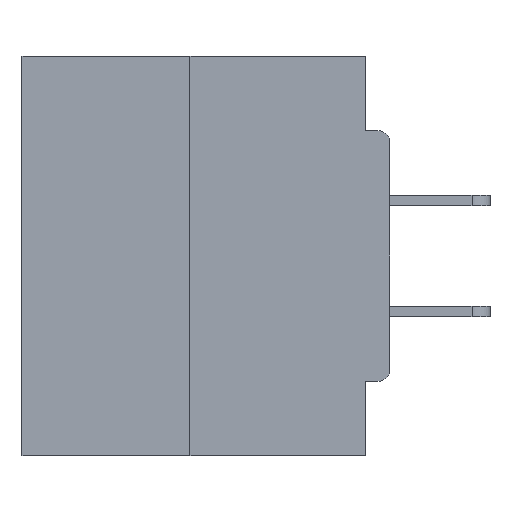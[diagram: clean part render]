
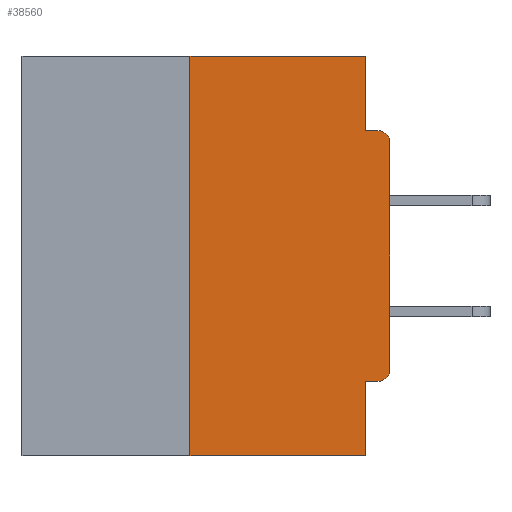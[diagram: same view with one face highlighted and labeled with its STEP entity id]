
A CAD part, left-side view. The second image highlights one B-rep face of the part: STEP entity #38560.
In plain terms, the highlighted planar face has unit normal (-1, 0, 0).
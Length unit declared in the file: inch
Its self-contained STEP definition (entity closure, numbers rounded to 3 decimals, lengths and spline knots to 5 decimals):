
#1169 = VERTEX_POINT ( 'NONE', #15668 ) ;
#1440 = CARTESIAN_POINT ( 'NONE',  ( 0., 0.25, 0. ) ) ;
#1769 = ORIENTED_EDGE ( 'NONE', *, *, #43550, .T. ) ;
#1906 = ORIENTED_EDGE ( 'NONE', *, *, #11319, .F. ) ;
#2708 = EDGE_CURVE ( 'NONE', #27769, #8198, #40876, .T. ) ;
#2900 = EDGE_CURVE ( 'NONE', #39610, #29801, #35509, .T. ) ;
#3965 = CARTESIAN_POINT ( 'NONE',  ( 0., 0.031, 0. ) ) ;
#4044 = DIRECTION ( 'NONE',  ( 1., 0., 0. ) ) ;
#4842 = LINE ( 'NONE', #8474, #19387 ) ;
#5030 = CARTESIAN_POINT ( 'NONE',  ( 0., 0.031, -0.5 ) ) ;
#5822 = VECTOR ( 'NONE', #8052, 39.37008 ) ;
#5872 = VERTEX_POINT ( 'NONE', #31267 ) ;
#6725 = EDGE_CURVE ( 'NONE', #26893, #35345, #37478, .T. ) ;
#8022 = DIRECTION ( 'NONE',  ( -1., 0., 0. ) ) ;
#8052 = DIRECTION ( 'NONE',  ( 0., 0., 1. ) ) ;
#8198 = VERTEX_POINT ( 'NONE', #33186 ) ;
#8277 = AXIS2_PLACEMENT_3D ( 'NONE', #28450, #4044, #28293 ) ;
#8474 = CARTESIAN_POINT ( 'NONE',  ( 0., 0.25, 0. ) ) ;
#8538 = VECTOR ( 'NONE', #15421, 39.37008 ) ;
#8597 = AXIS2_PLACEMENT_3D ( 'NONE', #35478, #8022, #11481 ) ;
#9036 = ORIENTED_EDGE ( 'NONE', *, *, #43108, .F. ) ;
#9143 = ORIENTED_EDGE ( 'NONE', *, *, #37754, .T. ) ;
#9298 = DIRECTION ( 'NONE',  ( 0., -1., 0. ) ) ;
#9304 = LINE ( 'NONE', #9726, #37368 ) ;
#9726 = CARTESIAN_POINT ( 'NONE',  ( 0., 0.46, -0.5 ) ) ;
#11319 = EDGE_CURVE ( 'NONE', #25590, #27769, #13968, .T. ) ;
#11481 = DIRECTION ( 'NONE',  ( 0., 0., -1. ) ) ;
#11743 = CARTESIAN_POINT ( 'NONE',  ( 0., 0.031, -0.4065 ) ) ;
#13191 = EDGE_CURVE ( 'NONE', #25590, #39610, #21374, .T. ) ;
#13324 = VECTOR ( 'NONE', #18516, 39.37008 ) ;
#13517 = DIRECTION ( 'NONE',  ( 0., 1., 0. ) ) ;
#13968 = LINE ( 'NONE', #31444, #34471 ) ;
#15421 = DIRECTION ( 'NONE',  ( 0., 0., -1. ) ) ;
#15668 = CARTESIAN_POINT ( 'NONE',  ( 0., 0.25, -0.5 ) ) ;
#16754 = EDGE_CURVE ( 'NONE', #5872, #30201, #39963, .T. ) ;
#16785 = CARTESIAN_POINT ( 'NONE',  ( 0., 0.015, -0.4065 ) ) ;
#17916 = PLANE ( 'NONE',  #8277 ) ;
#18516 = DIRECTION ( 'NONE',  ( 0., 0., -1. ) ) ;
#18864 = DIRECTION ( 'NONE',  ( 0., 0., 1. ) ) ;
#18934 = FACE_OUTER_BOUND ( 'NONE', #24641, .T. ) ;
#19387 = VECTOR ( 'NONE', #18864, 39.37008 ) ;
#21374 = CIRCLE ( 'NONE', #8597, 0.015 ) ;
#22225 = DIRECTION ( 'NONE',  ( 0., -1., 0. ) ) ;
#23190 = ORIENTED_EDGE ( 'NONE', *, *, #6725, .F. ) ;
#23720 = CARTESIAN_POINT ( 'NONE',  ( 0., 0.015, -0.1085 ) ) ;
#24641 = EDGE_LOOP ( 'NONE', ( #23190, #32181, #9143, #34505, #1906, #27550, #33647, #1769, #42073, #9036 ) ) ;
#24978 = CARTESIAN_POINT ( 'NONE',  ( 0., 0.46, 0. ) ) ;
#25590 = VERTEX_POINT ( 'NONE', #16785 ) ;
#26653 = VECTOR ( 'NONE', #31737, 39.37008 ) ;
#26893 = VERTEX_POINT ( 'NONE', #1440 ) ;
#27550 = ORIENTED_EDGE ( 'NONE', *, *, #13191, .T. ) ;
#27769 = VERTEX_POINT ( 'NONE', #11743 ) ;
#28293 = DIRECTION ( 'NONE',  ( 0., 0., -1. ) ) ;
#28450 = CARTESIAN_POINT ( 'NONE',  ( 0., 0.46, 0. ) ) ;
#28613 = AXIS2_PLACEMENT_3D ( 'NONE', #23720, #39744, #34315 ) ;
#28708 = CARTESIAN_POINT ( 'NONE',  ( 0., 0., 0. ) ) ;
#28907 = CARTESIAN_POINT ( 'NONE',  ( 0., 0.031, 0. ) ) ;
#29158 = CARTESIAN_POINT ( 'NONE',  ( 0., 0.015, -0.0935 ) ) ;
#29801 = VERTEX_POINT ( 'NONE', #35452 ) ;
#30201 = VERTEX_POINT ( 'NONE', #29158 ) ;
#30813 = VECTOR ( 'NONE', #22225, 39.37008 ) ;
#31267 = CARTESIAN_POINT ( 'NONE',  ( 0., 0.031, -0.0935 ) ) ;
#31444 = CARTESIAN_POINT ( 'NONE',  ( 0., 0., -0.4065 ) ) ;
#31639 = LINE ( 'NONE', #28907, #13324 ) ;
#31737 = DIRECTION ( 'NONE',  ( 0., -1., 0. ) ) ;
#32181 = ORIENTED_EDGE ( 'NONE', *, *, #33854, .F. ) ;
#33186 = CARTESIAN_POINT ( 'NONE',  ( 0., 0.031, -0.5 ) ) ;
#33429 = CARTESIAN_POINT ( 'NONE',  ( 0., 0., -0.3915 ) ) ;
#33647 = ORIENTED_EDGE ( 'NONE', *, *, #2900, .T. ) ;
#33854 = EDGE_CURVE ( 'NONE', #1169, #26893, #4842, .T. ) ;
#34315 = DIRECTION ( 'NONE',  ( 0., 0., -1. ) ) ;
#34471 = VECTOR ( 'NONE', #13517, 39.37008 ) ;
#34505 = ORIENTED_EDGE ( 'NONE', *, *, #2708, .F. ) ;
#34776 = CIRCLE ( 'NONE', #28613, 0.015 ) ;
#35345 = VERTEX_POINT ( 'NONE', #3965 ) ;
#35452 = CARTESIAN_POINT ( 'NONE',  ( 0., 0., -0.1085 ) ) ;
#35478 = CARTESIAN_POINT ( 'NONE',  ( 0., 0.015, -0.3915 ) ) ;
#35509 = LINE ( 'NONE', #28708, #5822 ) ;
#37368 = VECTOR ( 'NONE', #9298, 39.37008 ) ;
#37478 = LINE ( 'NONE', #24978, #26653 ) ;
#37754 = EDGE_CURVE ( 'NONE', #1169, #8198, #9304, .T. ) ;
#38560 = ADVANCED_FACE ( 'NONE', ( #18934 ), #17916, .F. ) ;
#39610 = VERTEX_POINT ( 'NONE', #33429 ) ;
#39744 = DIRECTION ( 'NONE',  ( -1., 0., 0. ) ) ;
#39963 = LINE ( 'NONE', #42863, #30813 ) ;
#40876 = LINE ( 'NONE', #5030, #8538 ) ;
#42073 = ORIENTED_EDGE ( 'NONE', *, *, #16754, .F. ) ;
#42863 = CARTESIAN_POINT ( 'NONE',  ( 0., 0., -0.0935 ) ) ;
#43108 = EDGE_CURVE ( 'NONE', #35345, #5872, #31639, .T. ) ;
#43550 = EDGE_CURVE ( 'NONE', #29801, #30201, #34776, .T. ) ;
